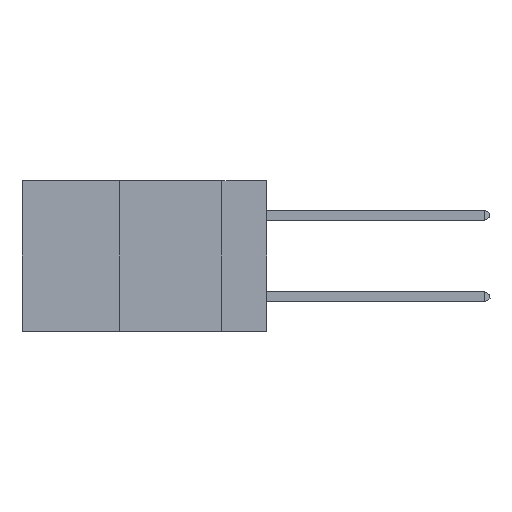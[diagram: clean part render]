
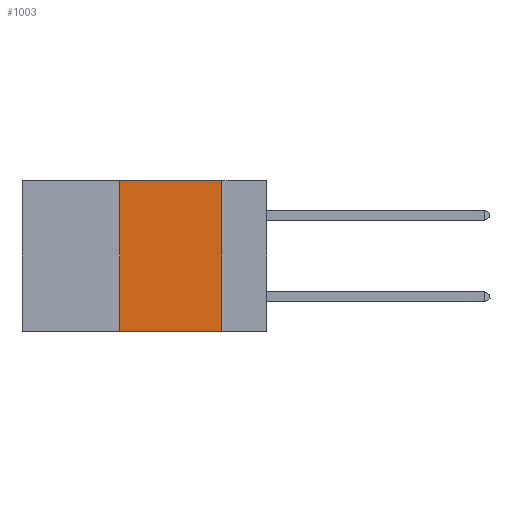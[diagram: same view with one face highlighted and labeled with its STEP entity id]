
A CAD part, left-side view. The second image highlights one B-rep face of the part: STEP entity #1003.
In plain terms, the highlighted planar face has unit normal (-1, 0, 0).
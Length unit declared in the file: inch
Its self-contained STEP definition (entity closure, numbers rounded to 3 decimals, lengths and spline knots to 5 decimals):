
#112 = DIRECTION ( 'NONE',  ( 0., 0., 1. ) ) ;
#273 = LINE ( 'NONE', #3825, #6178 ) ;
#371 = DIRECTION ( 'NONE',  ( 0., -1., 0. ) ) ;
#749 = PLANE ( 'NONE',  #6819 ) ;
#750 = ORIENTED_EDGE ( 'NONE', *, *, #6384, .F. ) ;
#1003 = ADVANCED_FACE ( 'NONE', ( #2825 ), #749, .F. ) ;
#1942 = CARTESIAN_POINT ( 'NONE',  ( 0., 0.11, 0. ) ) ;
#1952 = VECTOR ( 'NONE', #5491, 39.37008 ) ;
#2122 = CARTESIAN_POINT ( 'NONE',  ( 0., 0.36, 0. ) ) ;
#2388 = EDGE_LOOP ( 'NONE', ( #750, #5727, #5075, #3555 ) ) ;
#2482 = VERTEX_POINT ( 'NONE', #6713 ) ;
#2585 = EDGE_CURVE ( 'NONE', #5690, #8752, #3080, .T. ) ;
#2825 = FACE_OUTER_BOUND ( 'NONE', #2388, .T. ) ;
#2827 = CARTESIAN_POINT ( 'NONE',  ( 0., 0.6, 0. ) ) ;
#2845 = EDGE_CURVE ( 'NONE', #5690, #4439, #6543, .T. ) ;
#3080 = LINE ( 'NONE', #3871, #7191 ) ;
#3183 = DIRECTION ( 'NONE',  ( 0., -1., 0. ) ) ;
#3364 = CARTESIAN_POINT ( 'NONE',  ( 0., 0.36, -0.37 ) ) ;
#3555 = ORIENTED_EDGE ( 'NONE', *, *, #2585, .T. ) ;
#3781 = CARTESIAN_POINT ( 'NONE',  ( 0., 0.36, 0. ) ) ;
#3825 = CARTESIAN_POINT ( 'NONE',  ( 0., 0.6, 0. ) ) ;
#3871 = CARTESIAN_POINT ( 'NONE',  ( 0., 0.6, -0.37 ) ) ;
#3902 = EDGE_CURVE ( 'NONE', #4439, #2482, #273, .T. ) ;
#4254 = CARTESIAN_POINT ( 'NONE',  ( 0., 0.11, -0.37 ) ) ;
#4439 = VERTEX_POINT ( 'NONE', #3781 ) ;
#4994 = VECTOR ( 'NONE', #112, 39.37008 ) ;
#5075 = ORIENTED_EDGE ( 'NONE', *, *, #2845, .F. ) ;
#5491 = DIRECTION ( 'NONE',  ( 0., 0., -1. ) ) ;
#5647 = DIRECTION ( 'NONE',  ( 0., 0., -1. ) ) ;
#5690 = VERTEX_POINT ( 'NONE', #3364 ) ;
#5727 = ORIENTED_EDGE ( 'NONE', *, *, #3902, .F. ) ;
#6178 = VECTOR ( 'NONE', #371, 39.37008 ) ;
#6384 = EDGE_CURVE ( 'NONE', #2482, #8752, #6909, .T. ) ;
#6543 = LINE ( 'NONE', #2122, #4994 ) ;
#6713 = CARTESIAN_POINT ( 'NONE',  ( 0., 0.11, 0. ) ) ;
#6819 = AXIS2_PLACEMENT_3D ( 'NONE', #2827, #6982, #5647 ) ;
#6909 = LINE ( 'NONE', #1942, #1952 ) ;
#6982 = DIRECTION ( 'NONE',  ( 1., 0., 0. ) ) ;
#7191 = VECTOR ( 'NONE', #3183, 39.37008 ) ;
#8752 = VERTEX_POINT ( 'NONE', #4254 ) ;
